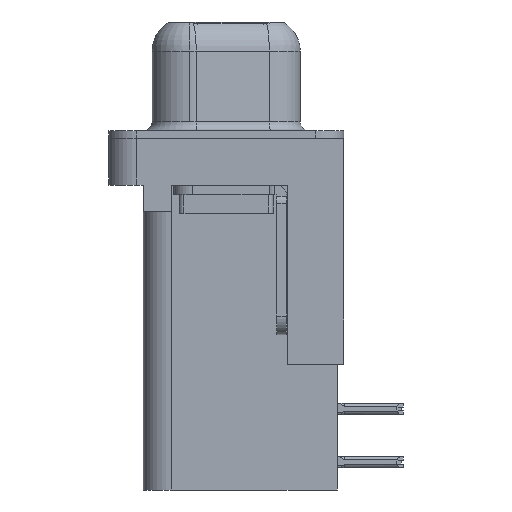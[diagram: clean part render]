
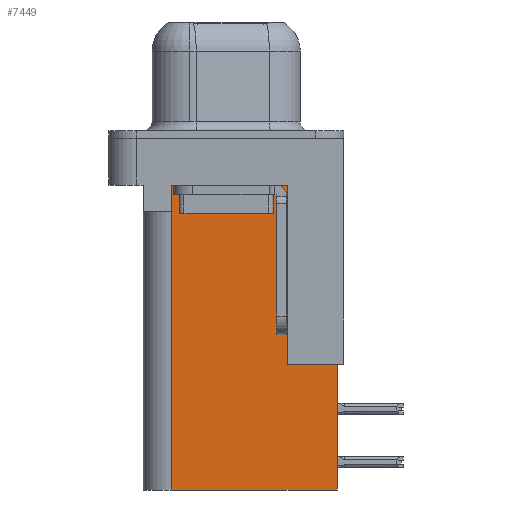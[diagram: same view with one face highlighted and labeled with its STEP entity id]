
A CAD part, left-side view. The second image highlights one B-rep face of the part: STEP entity #7449.
In plain terms, the highlighted planar face has unit normal (-1, 0, 0).
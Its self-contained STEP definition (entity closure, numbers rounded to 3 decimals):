
#104 = CARTESIAN_POINT ( 'NONE',  ( 3.79, 2.895, -3.9 ) ) ;
#541 = VERTEX_POINT ( 'NONE', #18262 ) ;
#629 = CARTESIAN_POINT ( 'NONE',  ( 3.79, 2.895, -2.5 ) ) ;
#1058 = CARTESIAN_POINT ( 'NONE',  ( 3.79, -5.925, -18.76 ) ) ;
#1074 = EDGE_CURVE ( 'NONE', #3648, #2145, #21468, .T. ) ;
#1677 = VECTOR ( 'NONE', #9777, 1000. ) ;
#1873 = VECTOR ( 'NONE', #10342, 1000. ) ;
#2145 = VERTEX_POINT ( 'NONE', #20753 ) ;
#2214 = DIRECTION ( 'NONE',  ( 0., 1., 0. ) ) ;
#2243 = VERTEX_POINT ( 'NONE', #1058 ) ;
#2269 = VERTEX_POINT ( 'NONE', #629 ) ;
#3207 = VECTOR ( 'NONE', #9053, 1000. ) ;
#3648 = VERTEX_POINT ( 'NONE', #14588 ) ;
#4497 = DIRECTION ( 'NONE',  ( 0., 1., 0. ) ) ;
#4915 = ORIENTED_EDGE ( 'NONE', *, *, #1074, .T. ) ;
#5275 = ORIENTED_EDGE ( 'NONE', *, *, #21063, .T. ) ;
#5385 = VERTEX_POINT ( 'NONE', #104 ) ;
#6054 = VECTOR ( 'NONE', #20866, 1000. ) ;
#6092 = LINE ( 'NONE', #11349, #1677 ) ;
#6395 = ORIENTED_EDGE ( 'NONE', *, *, #15846, .T. ) ;
#6560 = DIRECTION ( 'NONE',  ( 0., 1., 0. ) ) ;
#6579 = CARTESIAN_POINT ( 'NONE',  ( 3.79, -6.295, -12.05 ) ) ;
#6688 = FACE_OUTER_BOUND ( 'NONE', #8506, .T. ) ;
#7449 = ADVANCED_FACE ( 'NONE', ( #6688 ), #19833, .F. ) ;
#7705 = DIRECTION ( 'NONE',  ( 0., 0., -1. ) ) ;
#8506 = EDGE_LOOP ( 'NONE', ( #5275, #10077, #6395, #14506, #17829, #16753, #4915, #15499 ) ) ;
#8633 = CARTESIAN_POINT ( 'NONE',  ( 3.79, 2.925, -18.76 ) ) ;
#8834 = CARTESIAN_POINT ( 'NONE',  ( 3.79, 0., -3.9 ) ) ;
#9053 = DIRECTION ( 'NONE',  ( 0., 1., 0. ) ) ;
#9161 = CARTESIAN_POINT ( 'NONE',  ( 3.79, 2.895, -3.9 ) ) ;
#9777 = DIRECTION ( 'NONE',  ( 0., 1., 0. ) ) ;
#10045 = VECTOR ( 'NONE', #7705, 1000. ) ;
#10077 = ORIENTED_EDGE ( 'NONE', *, *, #20045, .T. ) ;
#10342 = DIRECTION ( 'NONE',  ( 0., 0., 1. ) ) ;
#10691 = DIRECTION ( 'NONE',  ( 0., 0., -1. ) ) ;
#10859 = VECTOR ( 'NONE', #10691, 1000. ) ;
#11007 = LINE ( 'NONE', #19236, #6054 ) ;
#11103 = CARTESIAN_POINT ( 'NONE',  ( 3.79, -3.295, -2.5 ) ) ;
#11345 = LINE ( 'NONE', #9161, #10859 ) ;
#11349 = CARTESIAN_POINT ( 'NONE',  ( 3.79, -3.295, -18.76 ) ) ;
#12375 = EDGE_CURVE ( 'NONE', #2145, #541, #11007, .T. ) ;
#12774 = LINE ( 'NONE', #8834, #16745 ) ;
#13201 = CARTESIAN_POINT ( 'NONE',  ( 3.79, -3.295, -18.76 ) ) ;
#13203 = EDGE_CURVE ( 'NONE', #13755, #18254, #15220, .T. ) ;
#13755 = VERTEX_POINT ( 'NONE', #8633 ) ;
#14506 = ORIENTED_EDGE ( 'NONE', *, *, #13203, .F. ) ;
#14521 = LINE ( 'NONE', #11103, #17911 ) ;
#14588 = CARTESIAN_POINT ( 'NONE',  ( 3.79, -5.925, -12.05 ) ) ;
#15220 = LINE ( 'NONE', #20334, #1873 ) ;
#15499 = ORIENTED_EDGE ( 'NONE', *, *, #12375, .T. ) ;
#15846 = EDGE_CURVE ( 'NONE', #5385, #18254, #12774, .T. ) ;
#16063 = CARTESIAN_POINT ( 'NONE',  ( 3.79, -5.925, -2. ) ) ;
#16607 = DIRECTION ( 'NONE',  ( 1., 0., 0. ) ) ;
#16745 = VECTOR ( 'NONE', #2214, 1000. ) ;
#16753 = ORIENTED_EDGE ( 'NONE', *, *, #21011, .F. ) ;
#17750 = AXIS2_PLACEMENT_3D ( 'NONE', #13201, #16607, #6560 ) ;
#17829 = ORIENTED_EDGE ( 'NONE', *, *, #21553, .F. ) ;
#17911 = VECTOR ( 'NONE', #4497, 1000. ) ;
#18254 = VERTEX_POINT ( 'NONE', #20256 ) ;
#18262 = CARTESIAN_POINT ( 'NONE',  ( 3.79, -3.295, -2.5 ) ) ;
#18970 = LINE ( 'NONE', #16063, #10045 ) ;
#19236 = CARTESIAN_POINT ( 'NONE',  ( 3.79, -3.295, -18.76 ) ) ;
#19833 = PLANE ( 'NONE',  #17750 ) ;
#20045 = EDGE_CURVE ( 'NONE', #2269, #5385, #11345, .T. ) ;
#20256 = CARTESIAN_POINT ( 'NONE',  ( 3.79, 2.925, -3.9 ) ) ;
#20334 = CARTESIAN_POINT ( 'NONE',  ( 3.79, 2.925, -18.76 ) ) ;
#20753 = CARTESIAN_POINT ( 'NONE',  ( 3.79, -3.295, -12.05 ) ) ;
#20866 = DIRECTION ( 'NONE',  ( 0., 0., 1. ) ) ;
#21011 = EDGE_CURVE ( 'NONE', #3648, #2243, #18970, .T. ) ;
#21063 = EDGE_CURVE ( 'NONE', #541, #2269, #14521, .T. ) ;
#21468 = LINE ( 'NONE', #6579, #3207 ) ;
#21553 = EDGE_CURVE ( 'NONE', #2243, #13755, #6092, .T. ) ;
